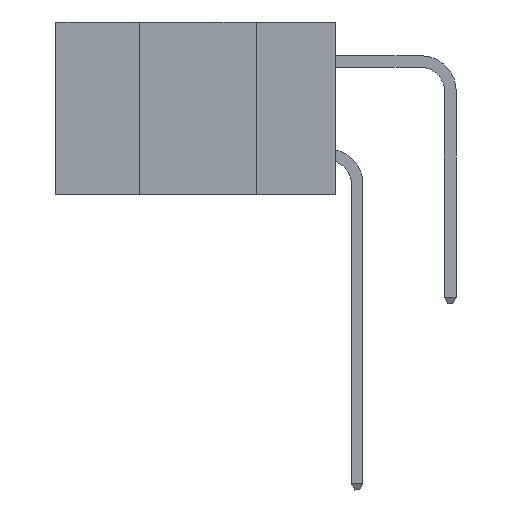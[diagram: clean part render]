
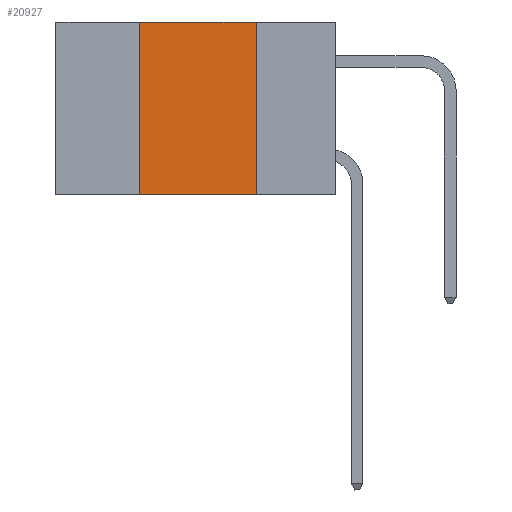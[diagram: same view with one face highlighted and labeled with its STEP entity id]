
A CAD part, left-side view. The second image highlights one B-rep face of the part: STEP entity #20927.
In plain terms, the highlighted planar face has unit normal (-1, 0, 0).
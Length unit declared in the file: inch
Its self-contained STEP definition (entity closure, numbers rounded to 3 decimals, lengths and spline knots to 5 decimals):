
#355 = ORIENTED_EDGE ( 'NONE', *, *, #12951, .F. ) ;
#491 = CARTESIAN_POINT ( 'NONE',  ( 0., 0.17, -0.37 ) ) ;
#898 = CARTESIAN_POINT ( 'NONE',  ( 0., 0.6, 0. ) ) ;
#1618 = DIRECTION ( 'NONE',  ( 0., -1., 0. ) ) ;
#1735 = LINE ( 'NONE', #9331, #10210 ) ;
#1826 = ORIENTED_EDGE ( 'NONE', *, *, #4266, .F. ) ;
#1965 = VERTEX_POINT ( 'NONE', #491 ) ;
#2573 = EDGE_CURVE ( 'NONE', #13355, #1965, #1735, .T. ) ;
#3311 = CARTESIAN_POINT ( 'NONE',  ( 0., 0.42, -0.37 ) ) ;
#3398 = CARTESIAN_POINT ( 'NONE',  ( 0., 0.6, 0. ) ) ;
#4266 = EDGE_CURVE ( 'NONE', #13355, #6523, #18455, .T. ) ;
#4882 = DIRECTION ( 'NONE',  ( 0., 0., -1. ) ) ;
#6523 = VERTEX_POINT ( 'NONE', #12310 ) ;
#6699 = DIRECTION ( 'NONE',  ( 0., -1., 0. ) ) ;
#7726 = AXIS2_PLACEMENT_3D ( 'NONE', #3398, #15334, #11490 ) ;
#9114 = LINE ( 'NONE', #9240, #17614 ) ;
#9240 = CARTESIAN_POINT ( 'NONE',  ( 0., 0.17, 0. ) ) ;
#9331 = CARTESIAN_POINT ( 'NONE',  ( 0., 0.6, -0.37 ) ) ;
#10210 = VECTOR ( 'NONE', #1618, 39.37008 ) ;
#10806 = VECTOR ( 'NONE', #23478, 39.37008 ) ;
#11490 = DIRECTION ( 'NONE',  ( 0., 0., -1. ) ) ;
#12310 = CARTESIAN_POINT ( 'NONE',  ( 0., 0.42, 0. ) ) ;
#12951 = EDGE_CURVE ( 'NONE', #14576, #1965, #9114, .T. ) ;
#13163 = FACE_OUTER_BOUND ( 'NONE', #14989, .T. ) ;
#13355 = VERTEX_POINT ( 'NONE', #3311 ) ;
#13812 = ORIENTED_EDGE ( 'NONE', *, *, #2573, .T. ) ;
#14407 = LINE ( 'NONE', #898, #19677 ) ;
#14576 = VERTEX_POINT ( 'NONE', #18653 ) ;
#14989 = EDGE_LOOP ( 'NONE', ( #355, #16779, #1826, #13812 ) ) ;
#15334 = DIRECTION ( 'NONE',  ( 1., 0., 0. ) ) ;
#16779 = ORIENTED_EDGE ( 'NONE', *, *, #23794, .F. ) ;
#17614 = VECTOR ( 'NONE', #4882, 39.37008 ) ;
#18455 = LINE ( 'NONE', #21404, #10806 ) ;
#18653 = CARTESIAN_POINT ( 'NONE',  ( 0., 0.17, 0. ) ) ;
#19677 = VECTOR ( 'NONE', #6699, 39.37008 ) ;
#20927 = ADVANCED_FACE ( 'NONE', ( #13163 ), #21022, .F. ) ;
#21022 = PLANE ( 'NONE',  #7726 ) ;
#21404 = CARTESIAN_POINT ( 'NONE',  ( 0., 0.42, 0. ) ) ;
#23478 = DIRECTION ( 'NONE',  ( 0., 0., 1. ) ) ;
#23794 = EDGE_CURVE ( 'NONE', #6523, #14576, #14407, .T. ) ;
